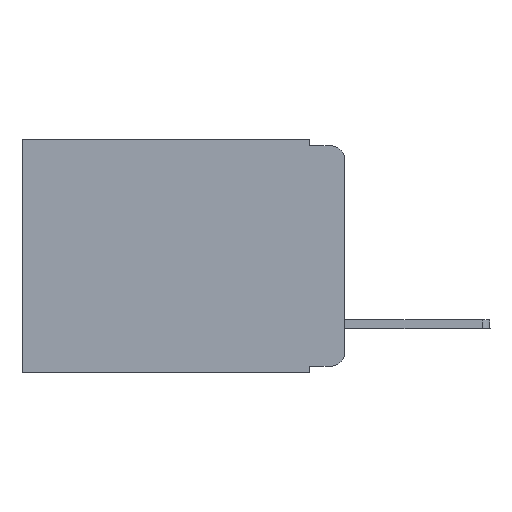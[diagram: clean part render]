
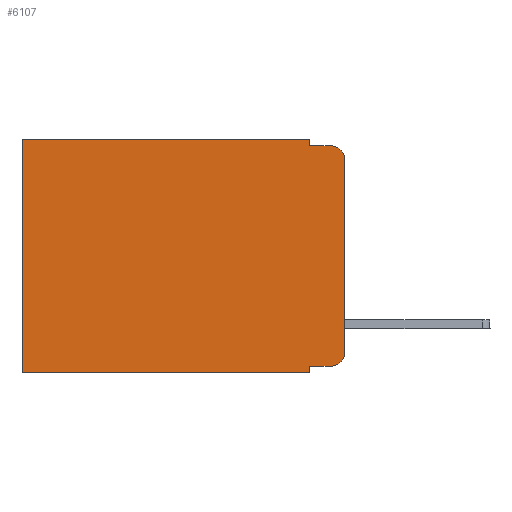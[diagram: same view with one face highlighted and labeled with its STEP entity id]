
A CAD part, left-side view. The second image highlights one B-rep face of the part: STEP entity #6107.
In plain terms, the highlighted planar face has unit normal (-1, 0, 0).
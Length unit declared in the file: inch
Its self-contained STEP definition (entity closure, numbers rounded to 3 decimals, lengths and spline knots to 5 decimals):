
#4 = ORIENTED_EDGE ( 'NONE', *, *, #11127, .F. ) ;
#80 = CARTESIAN_POINT ( 'NONE',  ( 0.298, 0., 0. ) ) ;
#183 = VECTOR ( 'NONE', #4133, 39.37008 ) ;
#214 = EDGE_CURVE ( 'NONE', #1435, #5513, #10974, .T. ) ;
#429 = CARTESIAN_POINT ( 'NONE',  ( 0.298, 0.051, -0.343 ) ) ;
#676 = EDGE_CURVE ( 'NONE', #4075, #10435, #10795, .T. ) ;
#1031 = ORIENTED_EDGE ( 'NONE', *, *, #9995, .T. ) ;
#1321 = AXIS2_PLACEMENT_3D ( 'NONE', #1437, #3612, #4686 ) ;
#1435 = VERTEX_POINT ( 'NONE', #3135 ) ;
#1437 = CARTESIAN_POINT ( 'NONE',  ( 0.298, 0., 0. ) ) ;
#1450 = DIRECTION ( 'NONE',  ( 0., 0., -1. ) ) ;
#1477 = ORIENTED_EDGE ( 'NONE', *, *, #214, .F. ) ;
#1526 = CARTESIAN_POINT ( 'NONE',  ( 0.298, 0., -0.343 ) ) ;
#1552 = EDGE_CURVE ( 'NONE', #4034, #10435, #13387, .T. ) ;
#1565 = LINE ( 'NONE', #9802, #8199 ) ;
#1624 = VERTEX_POINT ( 'NONE', #12823 ) ;
#2053 = AXIS2_PLACEMENT_3D ( 'NONE', #10847, #7876, #2536 ) ;
#2536 = DIRECTION ( 'NONE',  ( 0., 0., -1. ) ) ;
#2596 = LINE ( 'NONE', #1526, #13103 ) ;
#3063 = ORIENTED_EDGE ( 'NONE', *, *, #676, .F. ) ;
#3069 = FACE_OUTER_BOUND ( 'NONE', #8030, .T. ) ;
#3135 = CARTESIAN_POINT ( 'NONE',  ( 0.298, 0.051, 0. ) ) ;
#3612 = DIRECTION ( 'NONE',  ( 1., 0., 0. ) ) ;
#3671 = CARTESIAN_POINT ( 'NONE',  ( 0.298, 0.051, 0. ) ) ;
#4034 = VERTEX_POINT ( 'NONE', #6499 ) ;
#4075 = VERTEX_POINT ( 'NONE', #4762 ) ;
#4133 = DIRECTION ( 'NONE',  ( 0., 1., 0. ) ) ;
#4389 = DIRECTION ( 'NONE',  ( 0., 0., -1. ) ) ;
#4482 = ORIENTED_EDGE ( 'NONE', *, *, #8467, .F. ) ;
#4666 = ORIENTED_EDGE ( 'NONE', *, *, #5340, .T. ) ;
#4686 = DIRECTION ( 'NONE',  ( 0., 0., -1. ) ) ;
#4762 = CARTESIAN_POINT ( 'NONE',  ( 0.298, 0., -0.03 ) ) ;
#5101 = VERTEX_POINT ( 'NONE', #13464 ) ;
#5340 = EDGE_CURVE ( 'NONE', #1624, #5101, #1565, .T. ) ;
#5513 = VERTEX_POINT ( 'NONE', #6867 ) ;
#5924 = VECTOR ( 'NONE', #1450, 39.37008 ) ;
#6096 = EDGE_CURVE ( 'NONE', #4075, #8765, #6538, .T. ) ;
#6107 = ADVANCED_FACE ( 'NONE', ( #3069 ), #8942, .F. ) ;
#6341 = DIRECTION ( 'NONE',  ( 0., 0., -1. ) ) ;
#6392 = CARTESIAN_POINT ( 'NONE',  ( 0.298, 0.051, 0. ) ) ;
#6499 = CARTESIAN_POINT ( 'NONE',  ( 0.298, 0.02, -0.333 ) ) ;
#6538 = CIRCLE ( 'NONE', #2053, 0.02 ) ;
#6596 = CARTESIAN_POINT ( 'NONE',  ( 0.298, 0., -0.313 ) ) ;
#6760 = CARTESIAN_POINT ( 'NONE',  ( 0.298, 0.051, -0.333 ) ) ;
#6828 = CARTESIAN_POINT ( 'NONE',  ( 0.298, 0.02, -0.01 ) ) ;
#6867 = CARTESIAN_POINT ( 'NONE',  ( 0.298, 0.051, -0.01 ) ) ;
#6880 = VECTOR ( 'NONE', #9042, 39.37008 ) ;
#6976 = VECTOR ( 'NONE', #7032, 39.37008 ) ;
#7032 = DIRECTION ( 'NONE',  ( 0., -1., 0. ) ) ;
#7483 = CARTESIAN_POINT ( 'NONE',  ( 0.298, 0.051, -0.01 ) ) ;
#7730 = VECTOR ( 'NONE', #9978, 39.37008 ) ;
#7876 = DIRECTION ( 'NONE',  ( -1., 0., 0. ) ) ;
#7931 = EDGE_CURVE ( 'NONE', #5513, #8765, #9128, .T. ) ;
#8030 = EDGE_LOOP ( 'NONE', ( #3063, #13104, #10809, #1477, #9433, #4666, #4, #4482, #1031, #10604 ) ) ;
#8086 = CARTESIAN_POINT ( 'NONE',  ( 0.298, 0.02, -0.313 ) ) ;
#8199 = VECTOR ( 'NONE', #4389, 39.37008 ) ;
#8354 = VERTEX_POINT ( 'NONE', #10369 ) ;
#8467 = EDGE_CURVE ( 'NONE', #8354, #10985, #12702, .T. ) ;
#8765 = VERTEX_POINT ( 'NONE', #6828 ) ;
#8942 = PLANE ( 'NONE',  #1321 ) ;
#9042 = DIRECTION ( 'NONE',  ( 0., 0., -1. ) ) ;
#9128 = LINE ( 'NONE', #7483, #6976 ) ;
#9433 = ORIENTED_EDGE ( 'NONE', *, *, #12154, .T. ) ;
#9802 = CARTESIAN_POINT ( 'NONE',  ( 0.298, 0.473, 0. ) ) ;
#9978 = DIRECTION ( 'NONE',  ( 0., -1., 0. ) ) ;
#9995 = EDGE_CURVE ( 'NONE', #8354, #4034, #10680, .T. ) ;
#10209 = DIRECTION ( 'NONE',  ( -1., 0., 0. ) ) ;
#10303 = LINE ( 'NONE', #10412, #183 ) ;
#10369 = CARTESIAN_POINT ( 'NONE',  ( 0.298, 0.051, -0.333 ) ) ;
#10412 = CARTESIAN_POINT ( 'NONE',  ( 0.298, 0., 0. ) ) ;
#10413 = VECTOR ( 'NONE', #6341, 39.37008 ) ;
#10435 = VERTEX_POINT ( 'NONE', #6596 ) ;
#10604 = ORIENTED_EDGE ( 'NONE', *, *, #1552, .T. ) ;
#10680 = LINE ( 'NONE', #6760, #7730 ) ;
#10795 = LINE ( 'NONE', #80, #6880 ) ;
#10809 = ORIENTED_EDGE ( 'NONE', *, *, #7931, .F. ) ;
#10847 = CARTESIAN_POINT ( 'NONE',  ( 0.298, 0.02, -0.03 ) ) ;
#10883 = DIRECTION ( 'NONE',  ( 0., 1., 0. ) ) ;
#10974 = LINE ( 'NONE', #3671, #5924 ) ;
#10985 = VERTEX_POINT ( 'NONE', #429 ) ;
#11127 = EDGE_CURVE ( 'NONE', #10985, #5101, #2596, .T. ) ;
#11382 = AXIS2_PLACEMENT_3D ( 'NONE', #8086, #10209, #13345 ) ;
#12154 = EDGE_CURVE ( 'NONE', #1435, #1624, #10303, .T. ) ;
#12702 = LINE ( 'NONE', #6392, #10413 ) ;
#12823 = CARTESIAN_POINT ( 'NONE',  ( 0.298, 0.473, 0. ) ) ;
#13103 = VECTOR ( 'NONE', #10883, 39.37008 ) ;
#13104 = ORIENTED_EDGE ( 'NONE', *, *, #6096, .T. ) ;
#13345 = DIRECTION ( 'NONE',  ( 0., 0., -1. ) ) ;
#13387 = CIRCLE ( 'NONE', #11382, 0.02 ) ;
#13464 = CARTESIAN_POINT ( 'NONE',  ( 0.298, 0.473, -0.343 ) ) ;
